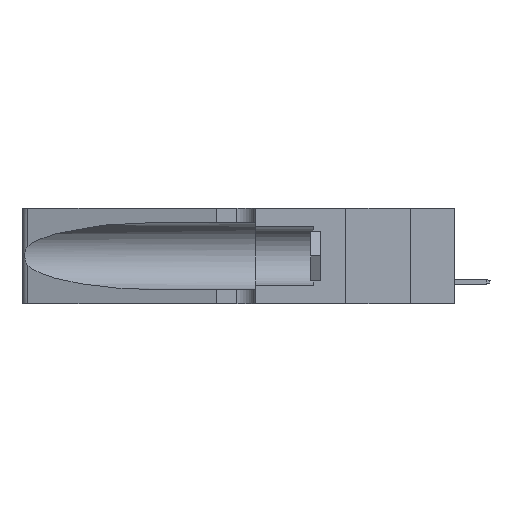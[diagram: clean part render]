
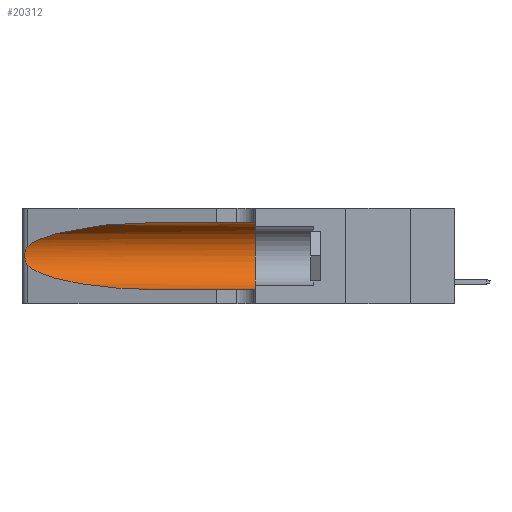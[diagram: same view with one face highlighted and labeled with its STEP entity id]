
A CAD part, left-side view. The second image highlights one B-rep face of the part: STEP entity #20312.
In plain terms, the highlighted cylindrical face has radius 3.308 mm (diameter 6.617 mm), a partial arc.
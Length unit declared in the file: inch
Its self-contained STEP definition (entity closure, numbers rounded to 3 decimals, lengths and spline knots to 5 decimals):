
#622 = CARTESIAN_POINT ( 'NONE',  ( 0.1305, 0.72297, 0.05475 ) ) ;
#3669 = VERTEX_POINT ( 'NONE', #26546 ) ;
#3687 = CARTESIAN_POINT ( 'NONE',  ( 0.1305, 1.61858, 0.05475 ) ) ;
#3832 = EDGE_CURVE ( 'NONE', #11033, #14453, #26132, .T. ) ;
#4323 = VERTEX_POINT ( 'NONE', #34399 ) ;
#4505 = CARTESIAN_POINT ( 'NONE',  ( 0.25555, 1.22994, 0.2215 ) ) ;
#5146 = CARTESIAN_POINT ( 'NONE',  ( 0.1305, 1.61858, 0.185 ) ) ;
#5811 = CARTESIAN_POINT ( 'NONE',  ( 0.25487, 1.22718, 0.14631 ) ) ;
#6541 = CARTESIAN_POINT ( 'NONE',  ( 0.2373, 1.15595, 0.28018 ) ) ;
#6734 = LINE ( 'NONE', #3687, #35872 ) ;
#7162 = CARTESIAN_POINT ( 'NONE',  ( 0.25487, 1.22718, 0.14631 ) ) ;
#7217 = CARTESIAN_POINT ( 'NONE',  ( 0.25487, 1.22718, 0.14631 ) ) ;
#9762 =( BOUNDED_CURVE ( )  B_SPLINE_CURVE ( 3, ( #12656, #16322, #6541, #18743 ),
 .UNSPECIFIED., .F., .T. ) 
 B_SPLINE_CURVE_WITH_KNOTS ( ( 4, 4 ),
 ( 1.5708, 2.84003 ),
 .UNSPECIFIED. ) 
 CURVE ( )  GEOMETRIC_REPRESENTATION_ITEM ( )  RATIONAL_B_SPLINE_CURVE ( ( 1., 0.87, 0.87, 1. ) ) 
 REPRESENTATION_ITEM ( '' )  );
#10610 = CARTESIAN_POINT ( 'NONE',  ( 0.25639, 1.23186, 0.15144 ) ) ;
#10809 = CARTESIAN_POINT ( 'NONE',  ( 0.25487, 1.22718, 0.22369 ) ) ;
#10985 = VERTEX_POINT ( 'NONE', #36683 ) ;
#11033 = VERTEX_POINT ( 'NONE', #5811 ) ;
#12415 = EDGE_CURVE ( 'NONE', #39243, #3669, #34855, .T. ) ;
#12656 = CARTESIAN_POINT ( 'NONE',  ( 0.1305, 0.72297, 0.31525 ) ) ;
#13325 = CARTESIAN_POINT ( 'NONE',  ( 0.1305, 0.72297, 0.05475 ) ) ;
#14140 = CIRCLE ( 'NONE', #36809, 0.13025 ) ;
#14453 = VERTEX_POINT ( 'NONE', #622 ) ;
#15958 = DIRECTION ( 'NONE',  ( 0., 0., 1. ) ) ;
#16322 = CARTESIAN_POINT ( 'NONE',  ( 0.18966, 0.96281, 0.31525 ) ) ;
#16642 = EDGE_CURVE ( 'NONE', #4323, #11033, #30203, .T. ) ;
#16780 = DIRECTION ( 'NONE',  ( 0., -1., 0. ) ) ;
#17548 = ORIENTED_EDGE ( 'NONE', *, *, #20467, .T. ) ;
#17563 = DIRECTION ( 'NONE',  ( 0., 0., -1. ) ) ;
#18743 = CARTESIAN_POINT ( 'NONE',  ( 0.25487, 1.22718, 0.22369 ) ) ;
#18938 = DIRECTION ( 'NONE',  ( 0., -1., 0. ) ) ;
#19846 = VECTOR ( 'NONE', #16780, 39.37008 ) ;
#20312 = ADVANCED_FACE ( 'NONE', ( #27073 ), #24045, .F. ) ;
#20467 = EDGE_CURVE ( 'NONE', #39243, #4323, #9762, .T. ) ;
#22046 = CARTESIAN_POINT ( 'NONE',  ( 0.1305, 0.35, 0.185 ) ) ;
#22604 = CARTESIAN_POINT ( 'NONE',  ( 0.26018, 1.23835, 0.19895 ) ) ;
#22808 = CARTESIAN_POINT ( 'NONE',  ( 0.25787, 1.23484, 0.2124 ) ) ;
#23002 = CARTESIAN_POINT ( 'NONE',  ( 0.25639, 1.23184, 0.21858 ) ) ;
#24045 = CYLINDRICAL_SURFACE ( 'NONE', #25259, 0.13025 ) ;
#24865 = ORIENTED_EDGE ( 'NONE', *, *, #29664, .T. ) ;
#24868 = DIRECTION ( 'NONE',  ( 0., 1., 0. ) ) ;
#25259 = AXIS2_PLACEMENT_3D ( 'NONE', #5146, #36812, #17563 ) ;
#25432 = CARTESIAN_POINT ( 'NONE',  ( 0.25555, 1.22993, 0.14849 ) ) ;
#25702 = CARTESIAN_POINT ( 'NONE',  ( 0.2373, 1.15595, 0.08982 ) ) ;
#26132 =( BOUNDED_CURVE ( )  B_SPLINE_CURVE ( 3, ( #7217, #25702, #38086, #13325 ),
 .UNSPECIFIED., .F., .T. ) 
 B_SPLINE_CURVE_WITH_KNOTS ( ( 4, 4 ),
 ( 3.44316, 4.71239 ),
 .UNSPECIFIED. ) 
 CURVE ( )  GEOMETRIC_REPRESENTATION_ITEM ( )  RATIONAL_B_SPLINE_CURVE ( ( 1., 0.87, 0.87, 1. ) ) 
 REPRESENTATION_ITEM ( '' )  );
#26546 = CARTESIAN_POINT ( 'NONE',  ( 0.1305, 0.35, 0.31525 ) ) ;
#27073 = FACE_OUTER_BOUND ( 'NONE', #39699, .T. ) ;
#29664 = EDGE_CURVE ( 'NONE', #14453, #10985, #6734, .T. ) ;
#30203 = B_SPLINE_CURVE_WITH_KNOTS ( 'NONE', 3,
 ( #10809, #4505, #23002, #22808, #38032, #22604, #34985, #35576, #35382, #32141, #35182, #10610, #25432, #7162 ),
 .UNSPECIFIED., .F., .F.,
 ( 4, 2, 2, 2, 2, 2, 4 ),
 ( 0., 0.00027, 0.00053, 0.00107, 0.0016, 0.00187, 0.00214 ),
 .UNSPECIFIED. ) ;
#31614 = CARTESIAN_POINT ( 'NONE',  ( 0.1305, 1.61858, 0.31525 ) ) ;
#32141 = CARTESIAN_POINT ( 'NONE',  ( 0.25856, 1.23593, 0.16098 ) ) ;
#32383 = ORIENTED_EDGE ( 'NONE', *, *, #12415, .F. ) ;
#33446 = ORIENTED_EDGE ( 'NONE', *, *, #39867, .F. ) ;
#33664 = CARTESIAN_POINT ( 'NONE',  ( 0.1305, 0.72297, 0.31525 ) ) ;
#34399 = CARTESIAN_POINT ( 'NONE',  ( 0.25487, 1.22718, 0.22369 ) ) ;
#34855 = LINE ( 'NONE', #31614, #19846 ) ;
#34985 = CARTESIAN_POINT ( 'NONE',  ( 0.26075, 1.23896, 0.19203 ) ) ;
#35182 = CARTESIAN_POINT ( 'NONE',  ( 0.25789, 1.23486, 0.15765 ) ) ;
#35339 = ORIENTED_EDGE ( 'NONE', *, *, #16642, .T. ) ;
#35382 = CARTESIAN_POINT ( 'NONE',  ( 0.26017, 1.23833, 0.17102 ) ) ;
#35411 = ORIENTED_EDGE ( 'NONE', *, *, #3832, .T. ) ;
#35576 = CARTESIAN_POINT ( 'NONE',  ( 0.26075, 1.23896, 0.178 ) ) ;
#35872 = VECTOR ( 'NONE', #18938, 39.37008 ) ;
#36683 = CARTESIAN_POINT ( 'NONE',  ( 0.1305, 0.35, 0.05475 ) ) ;
#36809 = AXIS2_PLACEMENT_3D ( 'NONE', #22046, #24868, #15958 ) ;
#36812 = DIRECTION ( 'NONE',  ( 0., -1., 0. ) ) ;
#38032 = CARTESIAN_POINT ( 'NONE',  ( 0.25854, 1.2359, 0.20912 ) ) ;
#38086 = CARTESIAN_POINT ( 'NONE',  ( 0.18966, 0.96281, 0.05475 ) ) ;
#39243 = VERTEX_POINT ( 'NONE', #33664 ) ;
#39699 = EDGE_LOOP ( 'NONE', ( #17548, #35339, #35411, #24865, #33446, #32383 ) ) ;
#39867 = EDGE_CURVE ( 'NONE', #3669, #10985, #14140, .T. ) ;
